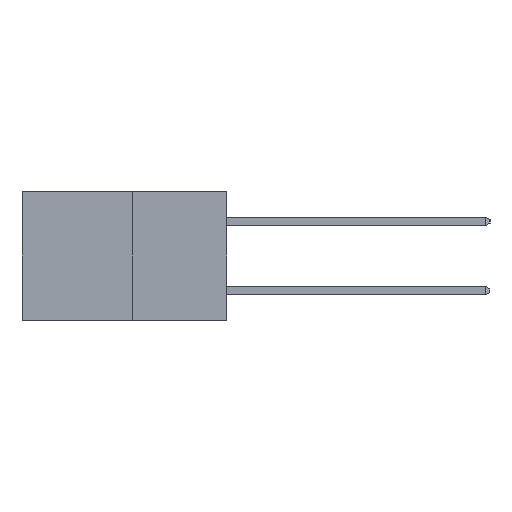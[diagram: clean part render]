
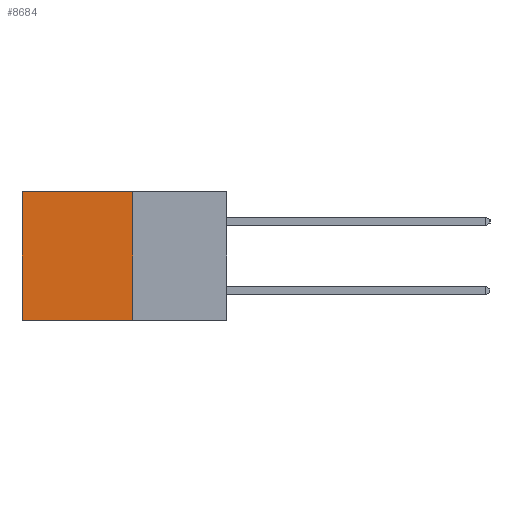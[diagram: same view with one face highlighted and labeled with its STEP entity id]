
A CAD part, left-side view. The second image highlights one B-rep face of the part: STEP entity #8684.
In plain terms, the highlighted planar face has unit normal (-1, 0, 0).
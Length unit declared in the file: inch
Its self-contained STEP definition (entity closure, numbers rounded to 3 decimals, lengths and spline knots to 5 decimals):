
#116 = FACE_OUTER_BOUND ( 'NONE', #6919, .T. ) ;
#898 = EDGE_CURVE ( 'NONE', #6569, #1002, #9988, .T. ) ;
#926 = EDGE_CURVE ( 'NONE', #3571, #6569, #9508, .T. ) ;
#1002 = VERTEX_POINT ( 'NONE', #7678 ) ;
#1340 = CARTESIAN_POINT ( 'NONE',  ( 0.277, 0.27, -0.37 ) ) ;
#1977 = VECTOR ( 'NONE', #9879, 39.37008 ) ;
#2366 = VECTOR ( 'NONE', #10400, 39.37008 ) ;
#2557 = CARTESIAN_POINT ( 'NONE',  ( 0.277, 0.27, -0.37 ) ) ;
#2635 = LINE ( 'NONE', #10810, #2366 ) ;
#2650 = VECTOR ( 'NONE', #10310, 39.37008 ) ;
#3557 = ORIENTED_EDGE ( 'NONE', *, *, #9290, .T. ) ;
#3571 = VERTEX_POINT ( 'NONE', #7886 ) ;
#4010 = ORIENTED_EDGE ( 'NONE', *, *, #7422, .T. ) ;
#4698 = AXIS2_PLACEMENT_3D ( 'NONE', #7690, #7675, #8414 ) ;
#5821 = VERTEX_POINT ( 'NONE', #6945 ) ;
#6569 = VERTEX_POINT ( 'NONE', #1340 ) ;
#6654 = ORIENTED_EDGE ( 'NONE', *, *, #926, .F. ) ;
#6919 = EDGE_LOOP ( 'NONE', ( #3557, #9967, #6654, #4010 ) ) ;
#6945 = CARTESIAN_POINT ( 'NONE',  ( 0.277, 0.59, 0. ) ) ;
#7091 = PLANE ( 'NONE',  #4698 ) ;
#7422 = EDGE_CURVE ( 'NONE', #3571, #5821, #2635, .T. ) ;
#7675 = DIRECTION ( 'NONE',  ( 1., 0., 0. ) ) ;
#7678 = CARTESIAN_POINT ( 'NONE',  ( 0.277, 0.59, -0.37 ) ) ;
#7690 = CARTESIAN_POINT ( 'NONE',  ( 0.277, 0.27, -0.37 ) ) ;
#7886 = CARTESIAN_POINT ( 'NONE',  ( 0.277, 0.27, 0. ) ) ;
#8009 = VECTOR ( 'NONE', #8308, 39.37008 ) ;
#8308 = DIRECTION ( 'NONE',  ( 0., 1., 0. ) ) ;
#8414 = DIRECTION ( 'NONE',  ( 0., 0., -1. ) ) ;
#8487 = CARTESIAN_POINT ( 'NONE',  ( 0.277, 0.27, -0.37 ) ) ;
#8684 = ADVANCED_FACE ( 'NONE', ( #116 ), #7091, .F. ) ;
#9095 = CARTESIAN_POINT ( 'NONE',  ( 0.277, 0.59, -0.37 ) ) ;
#9290 = EDGE_CURVE ( 'NONE', #5821, #1002, #10664, .T. ) ;
#9508 = LINE ( 'NONE', #2557, #2650 ) ;
#9879 = DIRECTION ( 'NONE',  ( 0., 0., -1. ) ) ;
#9967 = ORIENTED_EDGE ( 'NONE', *, *, #898, .F. ) ;
#9988 = LINE ( 'NONE', #8487, #8009 ) ;
#10310 = DIRECTION ( 'NONE',  ( 0., 0., -1. ) ) ;
#10400 = DIRECTION ( 'NONE',  ( 0., 1., 0. ) ) ;
#10664 = LINE ( 'NONE', #9095, #1977 ) ;
#10810 = CARTESIAN_POINT ( 'NONE',  ( 0.277, 0.27, 0. ) ) ;
